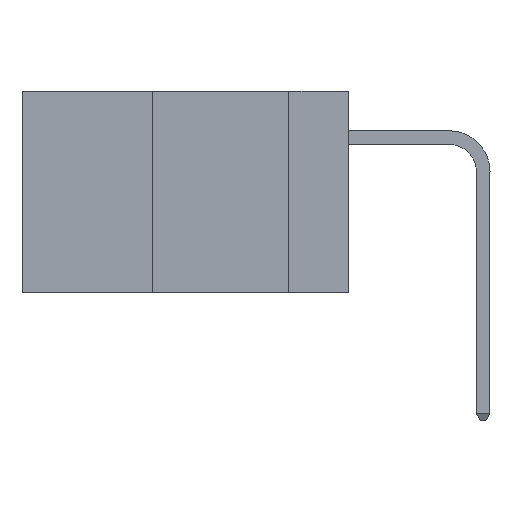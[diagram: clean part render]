
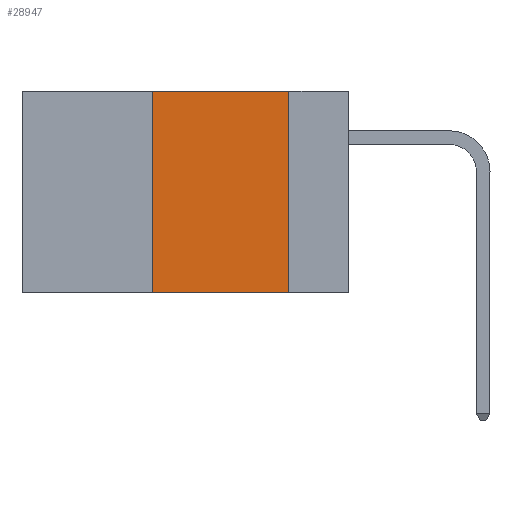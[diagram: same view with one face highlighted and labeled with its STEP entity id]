
A CAD part, left-side view. The second image highlights one B-rep face of the part: STEP entity #28947.
In plain terms, the highlighted planar face has unit normal (-1, 0, 0).
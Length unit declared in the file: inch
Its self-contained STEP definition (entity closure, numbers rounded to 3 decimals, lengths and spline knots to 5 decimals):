
#1152 = ORIENTED_EDGE ( 'NONE', *, *, #23414, .F. ) ;
#1419 = VERTEX_POINT ( 'NONE', #17905 ) ;
#3411 = EDGE_CURVE ( 'NONE', #27520, #1419, #22376, .T. ) ;
#3466 = CARTESIAN_POINT ( 'NONE',  ( 0., 0.6, 0. ) ) ;
#3954 = CARTESIAN_POINT ( 'NONE',  ( 0., 0.6, -0.37 ) ) ;
#4189 = ORIENTED_EDGE ( 'NONE', *, *, #30089, .T. ) ;
#4435 = DIRECTION ( 'NONE',  ( 0., 0., 1. ) ) ;
#9766 = VECTOR ( 'NONE', #12352, 39.37008 ) ;
#10353 = ORIENTED_EDGE ( 'NONE', *, *, #3411, .F. ) ;
#10906 = AXIS2_PLACEMENT_3D ( 'NONE', #3466, #31023, #28469 ) ;
#10951 = DIRECTION ( 'NONE',  ( 0., 0., -1. ) ) ;
#12352 = DIRECTION ( 'NONE',  ( 0., -1., 0. ) ) ;
#12560 = CARTESIAN_POINT ( 'NONE',  ( 0., 0.6, 0. ) ) ;
#12734 = CARTESIAN_POINT ( 'NONE',  ( 0., 0.11, 0. ) ) ;
#13618 = LINE ( 'NONE', #12560, #27593 ) ;
#14953 = VECTOR ( 'NONE', #4435, 39.37008 ) ;
#16155 = ORIENTED_EDGE ( 'NONE', *, *, #31769, .F. ) ;
#17366 = CARTESIAN_POINT ( 'NONE',  ( 0., 0.11, -0.37 ) ) ;
#17905 = CARTESIAN_POINT ( 'NONE',  ( 0., 0.36, 0. ) ) ;
#18790 = EDGE_LOOP ( 'NONE', ( #1152, #16155, #10353, #4189 ) ) ;
#18974 = VERTEX_POINT ( 'NONE', #12734 ) ;
#20043 = PLANE ( 'NONE',  #10906 ) ;
#20579 = LINE ( 'NONE', #21709, #27164 ) ;
#21709 = CARTESIAN_POINT ( 'NONE',  ( 0., 0.11, 0. ) ) ;
#22376 = LINE ( 'NONE', #26885, #14953 ) ;
#22437 = LINE ( 'NONE', #3954, #9766 ) ;
#23414 = EDGE_CURVE ( 'NONE', #18974, #29871, #20579, .T. ) ;
#23995 = FACE_OUTER_BOUND ( 'NONE', #18790, .T. ) ;
#26885 = CARTESIAN_POINT ( 'NONE',  ( 0., 0.36, 0. ) ) ;
#27164 = VECTOR ( 'NONE', #10951, 39.37008 ) ;
#27520 = VERTEX_POINT ( 'NONE', #28635 ) ;
#27593 = VECTOR ( 'NONE', #32428, 39.37008 ) ;
#28469 = DIRECTION ( 'NONE',  ( 0., 0., -1. ) ) ;
#28635 = CARTESIAN_POINT ( 'NONE',  ( 0., 0.36, -0.37 ) ) ;
#28947 = ADVANCED_FACE ( 'NONE', ( #23995 ), #20043, .F. ) ;
#29871 = VERTEX_POINT ( 'NONE', #17366 ) ;
#30089 = EDGE_CURVE ( 'NONE', #27520, #29871, #22437, .T. ) ;
#31023 = DIRECTION ( 'NONE',  ( 1., 0., 0. ) ) ;
#31769 = EDGE_CURVE ( 'NONE', #1419, #18974, #13618, .T. ) ;
#32428 = DIRECTION ( 'NONE',  ( 0., -1., 0. ) ) ;
